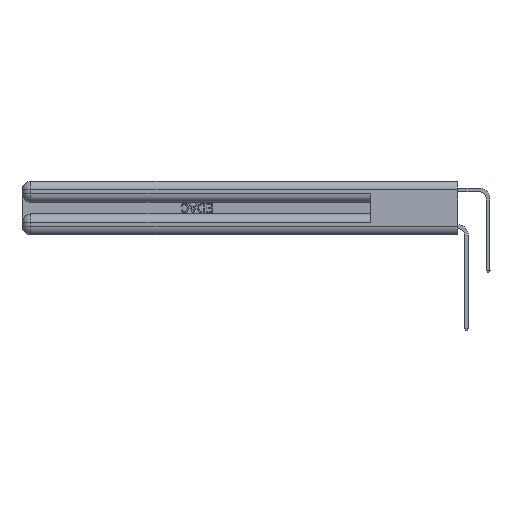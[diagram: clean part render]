
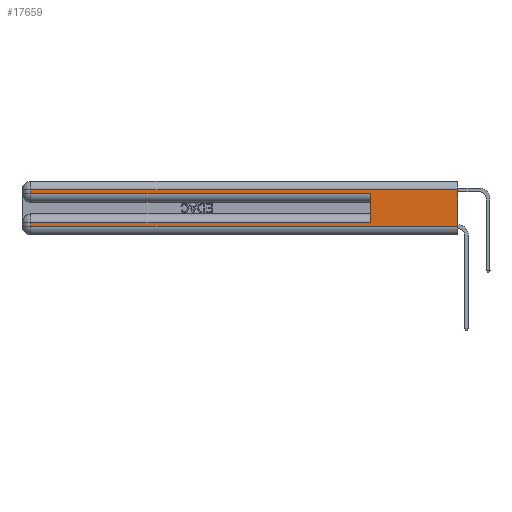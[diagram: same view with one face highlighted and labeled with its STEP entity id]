
A CAD part, left-side view. The second image highlights one B-rep face of the part: STEP entity #17659.
In plain terms, the highlighted planar face has unit normal (-1, 0, 0).
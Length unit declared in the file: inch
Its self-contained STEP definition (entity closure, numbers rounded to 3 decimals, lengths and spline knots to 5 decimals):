
#367 = EDGE_CURVE ( 'NONE', #33123, #25708, #30111, .T. ) ;
#1631 = CARTESIAN_POINT ( 'NONE',  ( 0., 0., 0.37 ) ) ;
#1802 = LINE ( 'NONE', #1631, #28746 ) ;
#1828 = CARTESIAN_POINT ( 'NONE',  ( 0., 0., 0.06 ) ) ;
#2025 = EDGE_CURVE ( 'NONE', #16642, #10508, #4496, .T. ) ;
#2308 = PLANE ( 'NONE',  #26987 ) ;
#2811 = EDGE_CURVE ( 'NONE', #25708, #16642, #12262, .T. ) ;
#3182 = LINE ( 'NONE', #3706, #18593 ) ;
#3569 = DIRECTION ( 'NONE',  ( 0., 0., 1. ) ) ;
#3706 = CARTESIAN_POINT ( 'NONE',  ( 0., 0., 0.285 ) ) ;
#3819 = EDGE_LOOP ( 'NONE', ( #26071, #31340, #30624, #33961, #20594, #28985, #12813, #12070 ) ) ;
#4496 = LINE ( 'NONE', #1828, #15541 ) ;
#6203 = CARTESIAN_POINT ( 'NONE',  ( 0., 0.6, 0.085 ) ) ;
#6682 = CARTESIAN_POINT ( 'NONE',  ( 0., 0.6, 0.285 ) ) ;
#6794 = EDGE_CURVE ( 'NONE', #25108, #27748, #22455, .T. ) ;
#7831 = DIRECTION ( 'NONE',  ( 0., 0., -1. ) ) ;
#7910 = DIRECTION ( 'NONE',  ( 0., 1., 0. ) ) ;
#8697 = VERTEX_POINT ( 'NONE', #6682 ) ;
#9361 = VECTOR ( 'NONE', #3569, 39.37008 ) ;
#9602 = VECTOR ( 'NONE', #7910, 39.37008 ) ;
#9755 = EDGE_CURVE ( 'NONE', #33123, #8697, #17143, .T. ) ;
#10508 = VERTEX_POINT ( 'NONE', #33361 ) ;
#12070 = ORIENTED_EDGE ( 'NONE', *, *, #2025, .T. ) ;
#12262 = LINE ( 'NONE', #26028, #33443 ) ;
#12813 = ORIENTED_EDGE ( 'NONE', *, *, #2811, .T. ) ;
#13212 = CARTESIAN_POINT ( 'NONE',  ( 0., 0., 0.37 ) ) ;
#13303 = VECTOR ( 'NONE', #32835, 39.37008 ) ;
#13524 = VERTEX_POINT ( 'NONE', #14531 ) ;
#14004 = CARTESIAN_POINT ( 'NONE',  ( 0., 0., 0.085 ) ) ;
#14531 = CARTESIAN_POINT ( 'NONE',  ( 0., 2.94, 0.285 ) ) ;
#15541 = VECTOR ( 'NONE', #26851, 39.37008 ) ;
#16642 = VERTEX_POINT ( 'NONE', #31285 ) ;
#17143 = LINE ( 'NONE', #28076, #9361 ) ;
#17659 = ADVANCED_FACE ( 'NONE', ( #26807 ), #2308, .F. ) ;
#18019 = CARTESIAN_POINT ( 'NONE',  ( 0., 2.94, 0.31 ) ) ;
#18593 = VECTOR ( 'NONE', #22493, 39.37008 ) ;
#19570 = DIRECTION ( 'NONE',  ( 0., 1., 0. ) ) ;
#19863 = EDGE_CURVE ( 'NONE', #27748, #13524, #27266, .T. ) ;
#20545 = EDGE_CURVE ( 'NONE', #25108, #10508, #1802, .T. ) ;
#20594 = ORIENTED_EDGE ( 'NONE', *, *, #9755, .F. ) ;
#22091 = CARTESIAN_POINT ( 'NONE',  ( 0., 0., 0.31 ) ) ;
#22455 = LINE ( 'NONE', #22091, #24080 ) ;
#22493 = DIRECTION ( 'NONE',  ( 0., -1., 0. ) ) ;
#22601 = CARTESIAN_POINT ( 'NONE',  ( 0., 2.94, 0.085 ) ) ;
#24080 = VECTOR ( 'NONE', #19570, 39.37008 ) ;
#24116 = DIRECTION ( 'NONE',  ( 1., 0., 0. ) ) ;
#24931 = CARTESIAN_POINT ( 'NONE',  ( 0., 2.94, 0.37 ) ) ;
#25108 = VERTEX_POINT ( 'NONE', #34129 ) ;
#25708 = VERTEX_POINT ( 'NONE', #22601 ) ;
#26028 = CARTESIAN_POINT ( 'NONE',  ( 0., 2.94, 0.37 ) ) ;
#26071 = ORIENTED_EDGE ( 'NONE', *, *, #20545, .F. ) ;
#26807 = FACE_OUTER_BOUND ( 'NONE', #3819, .T. ) ;
#26851 = DIRECTION ( 'NONE',  ( 0., -1., 0. ) ) ;
#26987 = AXIS2_PLACEMENT_3D ( 'NONE', #13212, #24116, #7831 ) ;
#27266 = LINE ( 'NONE', #24931, #13303 ) ;
#27748 = VERTEX_POINT ( 'NONE', #18019 ) ;
#28076 = CARTESIAN_POINT ( 'NONE',  ( 0., 0.6, 0.145 ) ) ;
#28746 = VECTOR ( 'NONE', #29158, 39.37008 ) ;
#28985 = ORIENTED_EDGE ( 'NONE', *, *, #367, .T. ) ;
#29158 = DIRECTION ( 'NONE',  ( 0., 0., -1. ) ) ;
#30111 = LINE ( 'NONE', #14004, #9602 ) ;
#30624 = ORIENTED_EDGE ( 'NONE', *, *, #19863, .T. ) ;
#31070 = DIRECTION ( 'NONE',  ( 0., 0., -1. ) ) ;
#31285 = CARTESIAN_POINT ( 'NONE',  ( 0., 2.94, 0.06 ) ) ;
#31340 = ORIENTED_EDGE ( 'NONE', *, *, #6794, .T. ) ;
#32835 = DIRECTION ( 'NONE',  ( 0., 0., -1. ) ) ;
#33006 = EDGE_CURVE ( 'NONE', #13524, #8697, #3182, .T. ) ;
#33123 = VERTEX_POINT ( 'NONE', #6203 ) ;
#33361 = CARTESIAN_POINT ( 'NONE',  ( 0., 0., 0.06 ) ) ;
#33443 = VECTOR ( 'NONE', #31070, 39.37008 ) ;
#33961 = ORIENTED_EDGE ( 'NONE', *, *, #33006, .T. ) ;
#34129 = CARTESIAN_POINT ( 'NONE',  ( 0., 0., 0.31 ) ) ;
